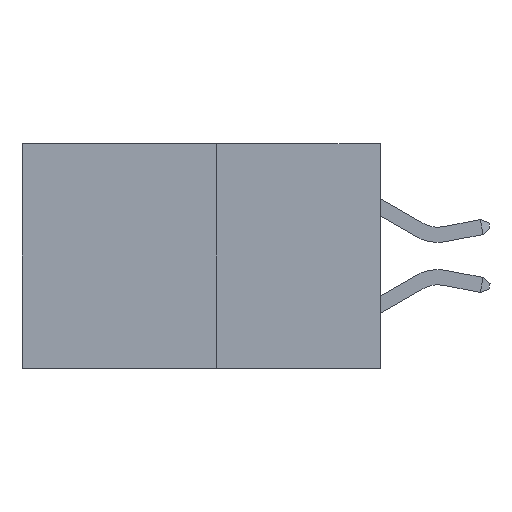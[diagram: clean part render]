
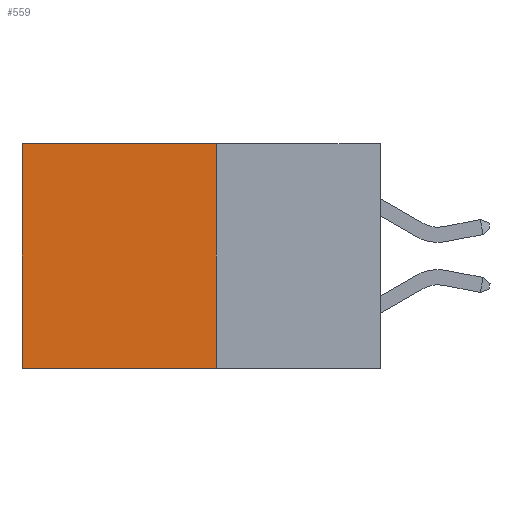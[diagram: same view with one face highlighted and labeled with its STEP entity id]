
A CAD part, left-side view. The second image highlights one B-rep face of the part: STEP entity #559.
In plain terms, the highlighted planar face has unit normal (-1, 0, 0).
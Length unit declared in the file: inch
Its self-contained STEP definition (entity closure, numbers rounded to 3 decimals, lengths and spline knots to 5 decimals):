
#559 = ADVANCED_FACE ( 'NONE', ( #3786 ), #1936, .F. ) ;
#1010 = EDGE_CURVE ( 'NONE', #10573, #8059, #5456, .T. ) ;
#1168 = VECTOR ( 'NONE', #10059, 39.37008 ) ;
#1240 = EDGE_CURVE ( 'NONE', #8059, #4927, #9890, .T. ) ;
#1745 = ORIENTED_EDGE ( 'NONE', *, *, #1240, .T. ) ;
#1856 = ORIENTED_EDGE ( 'NONE', *, *, #4229, .F. ) ;
#1873 = ORIENTED_EDGE ( 'NONE', *, *, #4767, .F. ) ;
#1936 = PLANE ( 'NONE',  #10424 ) ;
#2019 = ORIENTED_EDGE ( 'NONE', *, *, #1010, .T. ) ;
#2394 = VECTOR ( 'NONE', #8415, 39.37008 ) ;
#2596 = VERTEX_POINT ( 'NONE', #9105 ) ;
#3008 = CARTESIAN_POINT ( 'NONE',  ( 0.277, 0.27, 0. ) ) ;
#3258 = CARTESIAN_POINT ( 'NONE',  ( 0.277, 0.59, -0.37 ) ) ;
#3786 = FACE_OUTER_BOUND ( 'NONE', #10505, .T. ) ;
#3897 = VECTOR ( 'NONE', #5659, 39.37008 ) ;
#4229 = EDGE_CURVE ( 'NONE', #2596, #4927, #8950, .T. ) ;
#4395 = DIRECTION ( 'NONE',  ( 1., 0., 0. ) ) ;
#4481 = DIRECTION ( 'NONE',  ( 0., 0., -1. ) ) ;
#4767 = EDGE_CURVE ( 'NONE', #10573, #2596, #6026, .T. ) ;
#4927 = VERTEX_POINT ( 'NONE', #3258 ) ;
#5456 = LINE ( 'NONE', #8689, #9257 ) ;
#5659 = DIRECTION ( 'NONE',  ( 0., 0., -1. ) ) ;
#6026 = LINE ( 'NONE', #10281, #1168 ) ;
#6316 = DIRECTION ( 'NONE',  ( 0., 1., 0. ) ) ;
#8059 = VERTEX_POINT ( 'NONE', #8781 ) ;
#8415 = DIRECTION ( 'NONE',  ( 0., 1., 0. ) ) ;
#8577 = CARTESIAN_POINT ( 'NONE',  ( 0.277, 0.27, -0.37 ) ) ;
#8689 = CARTESIAN_POINT ( 'NONE',  ( 0.277, 0.27, 0. ) ) ;
#8781 = CARTESIAN_POINT ( 'NONE',  ( 0.277, 0.59, 0. ) ) ;
#8950 = LINE ( 'NONE', #8577, #2394 ) ;
#9105 = CARTESIAN_POINT ( 'NONE',  ( 0.277, 0.27, -0.37 ) ) ;
#9257 = VECTOR ( 'NONE', #6316, 39.37008 ) ;
#9890 = LINE ( 'NONE', #10555, #3897 ) ;
#9914 = CARTESIAN_POINT ( 'NONE',  ( 0.277, 0.27, -0.37 ) ) ;
#10059 = DIRECTION ( 'NONE',  ( 0., 0., -1. ) ) ;
#10281 = CARTESIAN_POINT ( 'NONE',  ( 0.277, 0.27, -0.37 ) ) ;
#10424 = AXIS2_PLACEMENT_3D ( 'NONE', #9914, #4395, #4481 ) ;
#10505 = EDGE_LOOP ( 'NONE', ( #1745, #1856, #1873, #2019 ) ) ;
#10555 = CARTESIAN_POINT ( 'NONE',  ( 0.277, 0.59, -0.37 ) ) ;
#10573 = VERTEX_POINT ( 'NONE', #3008 ) ;
